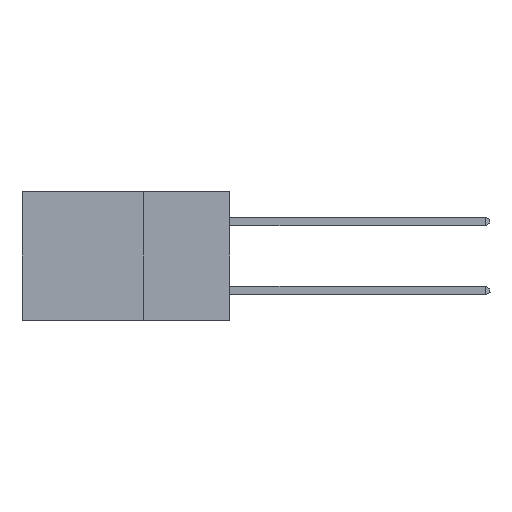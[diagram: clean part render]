
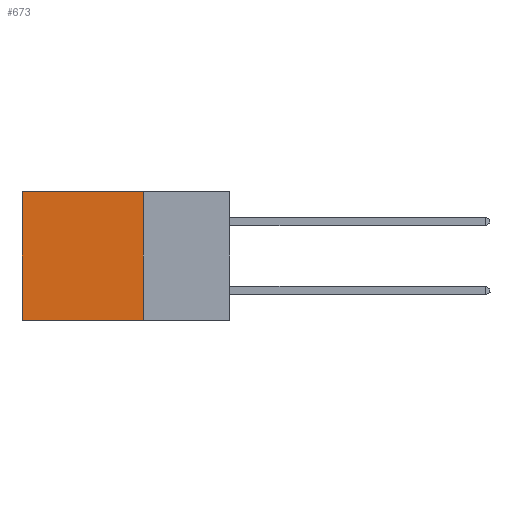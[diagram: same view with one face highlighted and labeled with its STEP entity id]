
A CAD part, left-side view. The second image highlights one B-rep face of the part: STEP entity #673.
In plain terms, the highlighted planar face has unit normal (-1, 0, 0).
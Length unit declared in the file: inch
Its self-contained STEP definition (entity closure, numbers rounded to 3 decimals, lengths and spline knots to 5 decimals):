
#673 = ADVANCED_FACE ( 'NONE', ( #6952 ), #19892, .F. ) ;
#1877 = CARTESIAN_POINT ( 'NONE',  ( 0.298, 0.6, -0.37 ) ) ;
#1921 = VERTEX_POINT ( 'NONE', #21591 ) ;
#3467 = EDGE_CURVE ( 'NONE', #7310, #20581, #23346, .T. ) ;
#3682 = VECTOR ( 'NONE', #4899, 39.37008 ) ;
#3961 = LINE ( 'NONE', #12998, #23632 ) ;
#4665 = CARTESIAN_POINT ( 'NONE',  ( 0.298, 0.25, 0. ) ) ;
#4899 = DIRECTION ( 'NONE',  ( 0., 0., -1. ) ) ;
#5488 = LINE ( 'NONE', #9137, #9786 ) ;
#5507 = EDGE_CURVE ( 'NONE', #1921, #7310, #12988, .T. ) ;
#5542 = VERTEX_POINT ( 'NONE', #14568 ) ;
#5926 = ORIENTED_EDGE ( 'NONE', *, *, #13657, .F. ) ;
#6746 = ORIENTED_EDGE ( 'NONE', *, *, #15454, .F. ) ;
#6845 = DIRECTION ( 'NONE',  ( 1., 0., 0. ) ) ;
#6952 = FACE_OUTER_BOUND ( 'NONE', #22583, .T. ) ;
#7310 = VERTEX_POINT ( 'NONE', #8818 ) ;
#8818 = CARTESIAN_POINT ( 'NONE',  ( 0.298, 0.6, 0. ) ) ;
#9137 = CARTESIAN_POINT ( 'NONE',  ( 0.298, 0.25, 0. ) ) ;
#9473 = ORIENTED_EDGE ( 'NONE', *, *, #3467, .T. ) ;
#9786 = VECTOR ( 'NONE', #14540, 39.37008 ) ;
#12256 = DIRECTION ( 'NONE',  ( 0., 1., 0. ) ) ;
#12444 = VECTOR ( 'NONE', #12256, 39.37008 ) ;
#12988 = LINE ( 'NONE', #4665, #12444 ) ;
#12998 = CARTESIAN_POINT ( 'NONE',  ( 0.298, 0.25, -0.37 ) ) ;
#13076 = DIRECTION ( 'NONE',  ( 0., 1., 0. ) ) ;
#13657 = EDGE_CURVE ( 'NONE', #1921, #5542, #5488, .T. ) ;
#14353 = AXIS2_PLACEMENT_3D ( 'NONE', #22763, #6845, #15491 ) ;
#14540 = DIRECTION ( 'NONE',  ( 0., 0., -1. ) ) ;
#14568 = CARTESIAN_POINT ( 'NONE',  ( 0.298, 0.25, -0.37 ) ) ;
#15454 = EDGE_CURVE ( 'NONE', #5542, #20581, #3961, .T. ) ;
#15491 = DIRECTION ( 'NONE',  ( 0., 0., -1. ) ) ;
#19022 = ORIENTED_EDGE ( 'NONE', *, *, #5507, .T. ) ;
#19259 = CARTESIAN_POINT ( 'NONE',  ( 0.298, 0.6, 0. ) ) ;
#19892 = PLANE ( 'NONE',  #14353 ) ;
#20581 = VERTEX_POINT ( 'NONE', #1877 ) ;
#21591 = CARTESIAN_POINT ( 'NONE',  ( 0.298, 0.25, 0. ) ) ;
#22583 = EDGE_LOOP ( 'NONE', ( #9473, #6746, #5926, #19022 ) ) ;
#22763 = CARTESIAN_POINT ( 'NONE',  ( 0.298, 0.25, 0. ) ) ;
#23346 = LINE ( 'NONE', #19259, #3682 ) ;
#23632 = VECTOR ( 'NONE', #13076, 39.37008 ) ;
